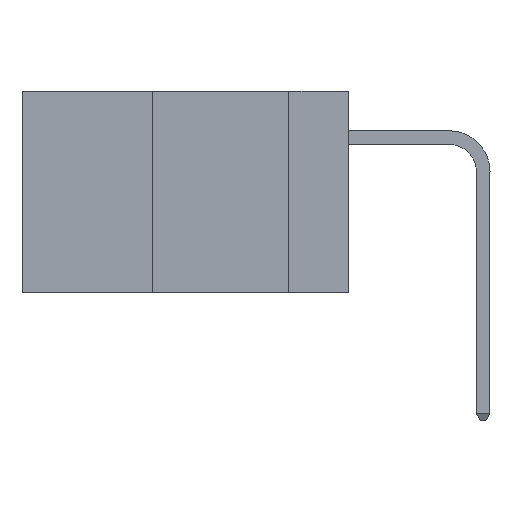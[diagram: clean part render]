
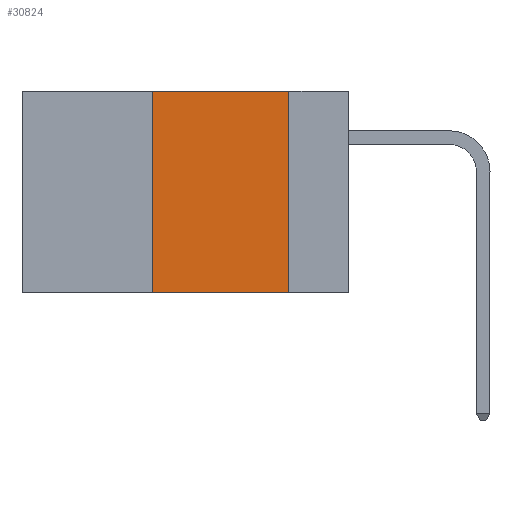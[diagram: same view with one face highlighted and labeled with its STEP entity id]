
A CAD part, left-side view. The second image highlights one B-rep face of the part: STEP entity #30824.
In plain terms, the highlighted planar face has unit normal (-1, 0, 0).
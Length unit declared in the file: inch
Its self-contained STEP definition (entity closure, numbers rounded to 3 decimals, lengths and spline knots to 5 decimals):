
#1698 = ORIENTED_EDGE ( 'NONE', *, *, #23165, .T. ) ;
#2711 = DIRECTION ( 'NONE',  ( 0., 0., -1. ) ) ;
#3721 = CARTESIAN_POINT ( 'NONE',  ( 0., 0.6, 0. ) ) ;
#4062 = EDGE_CURVE ( 'NONE', #15539, #32899, #7217, .T. ) ;
#4518 = EDGE_CURVE ( 'NONE', #32899, #33842, #13949, .T. ) ;
#5358 = ORIENTED_EDGE ( 'NONE', *, *, #4518, .F. ) ;
#6196 = VERTEX_POINT ( 'NONE', #35564 ) ;
#6310 = VECTOR ( 'NONE', #23345, 39.37008 ) ;
#6631 = DIRECTION ( 'NONE',  ( 0., 0., -1. ) ) ;
#6750 = FACE_OUTER_BOUND ( 'NONE', #24517, .T. ) ;
#7179 = LINE ( 'NONE', #19833, #32201 ) ;
#7217 = LINE ( 'NONE', #14873, #6310 ) ;
#11278 = CARTESIAN_POINT ( 'NONE',  ( 0., 0.6, 0. ) ) ;
#12903 = ORIENTED_EDGE ( 'NONE', *, *, #31242, .F. ) ;
#13183 = CARTESIAN_POINT ( 'NONE',  ( 0., 0.6, -0.37 ) ) ;
#13949 = LINE ( 'NONE', #11278, #26190 ) ;
#14098 = DIRECTION ( 'NONE',  ( 0., -1., 0. ) ) ;
#14873 = CARTESIAN_POINT ( 'NONE',  ( 0., 0.36, 0. ) ) ;
#15121 = AXIS2_PLACEMENT_3D ( 'NONE', #3721, #23652, #6631 ) ;
#15184 = PLANE ( 'NONE',  #15121 ) ;
#15539 = VERTEX_POINT ( 'NONE', #19031 ) ;
#16006 = DIRECTION ( 'NONE',  ( 0., -1., 0. ) ) ;
#19031 = CARTESIAN_POINT ( 'NONE',  ( 0., 0.36, -0.37 ) ) ;
#19833 = CARTESIAN_POINT ( 'NONE',  ( 0., 0.11, 0. ) ) ;
#22530 = CARTESIAN_POINT ( 'NONE',  ( 0., 0.36, 0. ) ) ;
#22755 = LINE ( 'NONE', #13183, #23609 ) ;
#23165 = EDGE_CURVE ( 'NONE', #15539, #6196, #22755, .T. ) ;
#23345 = DIRECTION ( 'NONE',  ( 0., 0., 1. ) ) ;
#23609 = VECTOR ( 'NONE', #16006, 39.37008 ) ;
#23652 = DIRECTION ( 'NONE',  ( 1., 0., 0. ) ) ;
#24517 = EDGE_LOOP ( 'NONE', ( #12903, #5358, #30905, #1698 ) ) ;
#26190 = VECTOR ( 'NONE', #14098, 39.37008 ) ;
#30824 = ADVANCED_FACE ( 'NONE', ( #6750 ), #15184, .F. ) ;
#30905 = ORIENTED_EDGE ( 'NONE', *, *, #4062, .F. ) ;
#31242 = EDGE_CURVE ( 'NONE', #33842, #6196, #7179, .T. ) ;
#32201 = VECTOR ( 'NONE', #2711, 39.37008 ) ;
#32899 = VERTEX_POINT ( 'NONE', #22530 ) ;
#33842 = VERTEX_POINT ( 'NONE', #34128 ) ;
#34128 = CARTESIAN_POINT ( 'NONE',  ( 0., 0.11, 0. ) ) ;
#35564 = CARTESIAN_POINT ( 'NONE',  ( 0., 0.11, -0.37 ) ) ;
